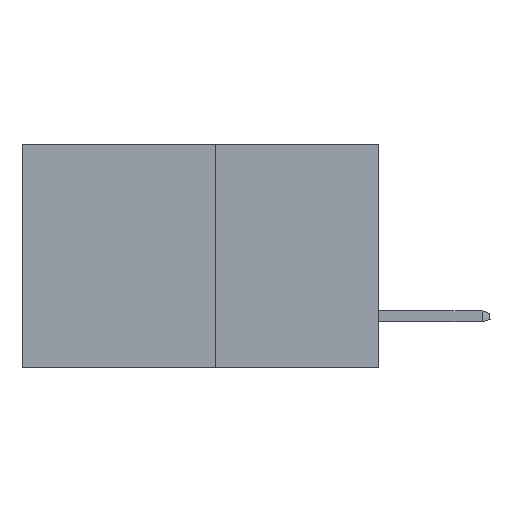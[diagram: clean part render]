
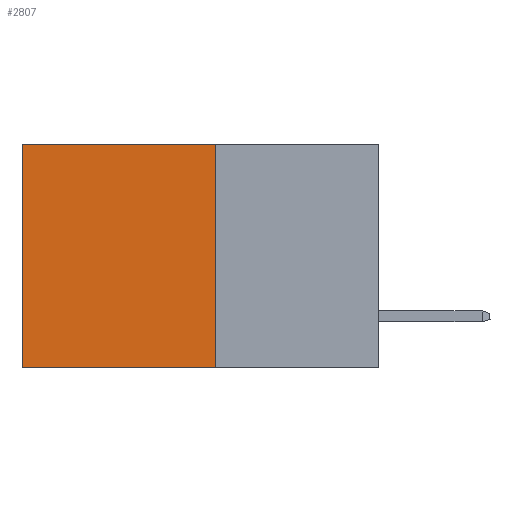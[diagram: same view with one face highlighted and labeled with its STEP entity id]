
A CAD part, left-side view. The second image highlights one B-rep face of the part: STEP entity #2807.
In plain terms, the highlighted planar face has unit normal (-1, 0, 0).
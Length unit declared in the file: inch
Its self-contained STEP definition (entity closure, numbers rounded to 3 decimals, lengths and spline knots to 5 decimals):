
#353 = CARTESIAN_POINT ( 'NONE',  ( 0.277, 0.27, 0. ) ) ;
#659 = VERTEX_POINT ( 'NONE', #8823 ) ;
#1859 = CARTESIAN_POINT ( 'NONE',  ( 0.277, 0.59, -0.37 ) ) ;
#1946 = LINE ( 'NONE', #14791, #15257 ) ;
#2807 = ADVANCED_FACE ( 'NONE', ( #5729 ), #16057, .F. ) ;
#2829 = ORIENTED_EDGE ( 'NONE', *, *, #10421, .T. ) ;
#2905 = EDGE_LOOP ( 'NONE', ( #2829, #8925, #5486, #4827 ) ) ;
#3140 = DIRECTION ( 'NONE',  ( 0., 1., 0. ) ) ;
#3638 = DIRECTION ( 'NONE',  ( 0., 0., -1. ) ) ;
#4087 = CARTESIAN_POINT ( 'NONE',  ( 0.277, 0.59, 0. ) ) ;
#4827 = ORIENTED_EDGE ( 'NONE', *, *, #11280, .T. ) ;
#5034 = AXIS2_PLACEMENT_3D ( 'NONE', #6115, #11198, #3638 ) ;
#5486 = ORIENTED_EDGE ( 'NONE', *, *, #13803, .F. ) ;
#5729 = FACE_OUTER_BOUND ( 'NONE', #2905, .T. ) ;
#5811 = LINE ( 'NONE', #10716, #8785 ) ;
#6115 = CARTESIAN_POINT ( 'NONE',  ( 0.277, 0.27, -0.37 ) ) ;
#6732 = EDGE_CURVE ( 'NONE', #8806, #9643, #5811, .T. ) ;
#7274 = CARTESIAN_POINT ( 'NONE',  ( 0.277, 0.27, -0.37 ) ) ;
#7320 = DIRECTION ( 'NONE',  ( 0., 0., -1. ) ) ;
#8238 = LINE ( 'NONE', #7274, #14463 ) ;
#8587 = DIRECTION ( 'NONE',  ( 0., 0., -1. ) ) ;
#8785 = VECTOR ( 'NONE', #3140, 39.37008 ) ;
#8806 = VERTEX_POINT ( 'NONE', #9202 ) ;
#8823 = CARTESIAN_POINT ( 'NONE',  ( 0.277, 0.27, 0. ) ) ;
#8925 = ORIENTED_EDGE ( 'NONE', *, *, #6732, .F. ) ;
#9070 = LINE ( 'NONE', #353, #15996 ) ;
#9202 = CARTESIAN_POINT ( 'NONE',  ( 0.277, 0.27, -0.37 ) ) ;
#9222 = DIRECTION ( 'NONE',  ( 0., 1., 0. ) ) ;
#9643 = VERTEX_POINT ( 'NONE', #1859 ) ;
#10421 = EDGE_CURVE ( 'NONE', #11249, #9643, #1946, .T. ) ;
#10716 = CARTESIAN_POINT ( 'NONE',  ( 0.277, 0.27, -0.37 ) ) ;
#11198 = DIRECTION ( 'NONE',  ( 1., 0., 0. ) ) ;
#11249 = VERTEX_POINT ( 'NONE', #4087 ) ;
#11280 = EDGE_CURVE ( 'NONE', #659, #11249, #9070, .T. ) ;
#13803 = EDGE_CURVE ( 'NONE', #659, #8806, #8238, .T. ) ;
#14463 = VECTOR ( 'NONE', #8587, 39.37008 ) ;
#14791 = CARTESIAN_POINT ( 'NONE',  ( 0.277, 0.59, -0.37 ) ) ;
#15257 = VECTOR ( 'NONE', #7320, 39.37008 ) ;
#15996 = VECTOR ( 'NONE', #9222, 39.37008 ) ;
#16057 = PLANE ( 'NONE',  #5034 ) ;
